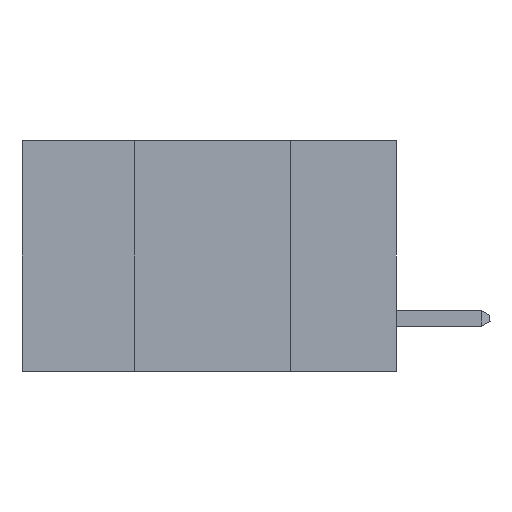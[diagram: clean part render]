
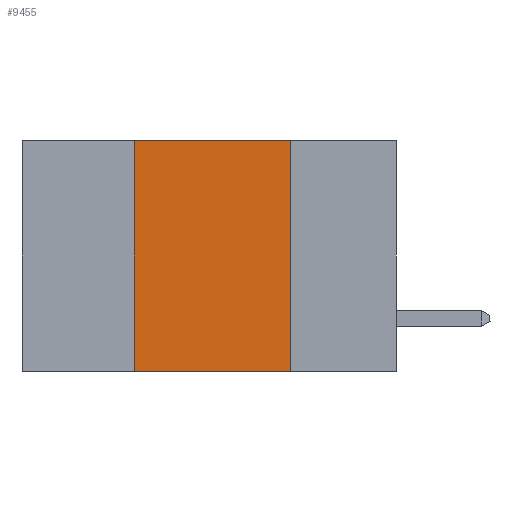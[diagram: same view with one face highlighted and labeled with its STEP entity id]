
A CAD part, left-side view. The second image highlights one B-rep face of the part: STEP entity #9455.
In plain terms, the highlighted planar face has unit normal (-1, 0, 0).
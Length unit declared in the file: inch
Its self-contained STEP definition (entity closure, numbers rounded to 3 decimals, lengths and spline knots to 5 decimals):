
#525 = CARTESIAN_POINT ( 'NONE',  ( 0., 0.17, 0. ) ) ;
#1495 = LINE ( 'NONE', #3169, #6757 ) ;
#2594 = DIRECTION ( 'NONE',  ( 0., 0., -1. ) ) ;
#2927 = CARTESIAN_POINT ( 'NONE',  ( 0., 0.42, -0.37 ) ) ;
#3167 = DIRECTION ( 'NONE',  ( 0., 0., -1. ) ) ;
#3169 = CARTESIAN_POINT ( 'NONE',  ( 0., 0.6, -0.37 ) ) ;
#3229 = AXIS2_PLACEMENT_3D ( 'NONE', #3696, #4717, #2594 ) ;
#3696 = CARTESIAN_POINT ( 'NONE',  ( 0., 0.6, 0. ) ) ;
#3770 = ORIENTED_EDGE ( 'NONE', *, *, #10901, .F. ) ;
#3911 = LINE ( 'NONE', #11110, #5869 ) ;
#4228 = DIRECTION ( 'NONE',  ( 0., -1., 0. ) ) ;
#4269 = CARTESIAN_POINT ( 'NONE',  ( 0., 0.17, 0. ) ) ;
#4399 = VECTOR ( 'NONE', #5413, 39.37008 ) ;
#4717 = DIRECTION ( 'NONE',  ( 1., 0., 0. ) ) ;
#4893 = LINE ( 'NONE', #7437, #4399 ) ;
#5028 = ORIENTED_EDGE ( 'NONE', *, *, #7295, .F. ) ;
#5382 = VERTEX_POINT ( 'NONE', #8426 ) ;
#5413 = DIRECTION ( 'NONE',  ( 0., -1., 0. ) ) ;
#5467 = EDGE_LOOP ( 'NONE', ( #8746, #5028, #3770, #12187 ) ) ;
#5651 = VERTEX_POINT ( 'NONE', #5855 ) ;
#5855 = CARTESIAN_POINT ( 'NONE',  ( 0., 0.17, -0.37 ) ) ;
#5869 = VECTOR ( 'NONE', #8908, 39.37008 ) ;
#6513 = LINE ( 'NONE', #4269, #6859 ) ;
#6757 = VECTOR ( 'NONE', #4228, 39.37008 ) ;
#6775 = PLANE ( 'NONE',  #3229 ) ;
#6859 = VECTOR ( 'NONE', #3167, 39.37008 ) ;
#7295 = EDGE_CURVE ( 'NONE', #5382, #12162, #4893, .T. ) ;
#7437 = CARTESIAN_POINT ( 'NONE',  ( 0., 0.6, 0. ) ) ;
#7615 = VERTEX_POINT ( 'NONE', #2927 ) ;
#8402 = FACE_OUTER_BOUND ( 'NONE', #5467, .T. ) ;
#8426 = CARTESIAN_POINT ( 'NONE',  ( 0., 0.42, 0. ) ) ;
#8746 = ORIENTED_EDGE ( 'NONE', *, *, #11843, .F. ) ;
#8908 = DIRECTION ( 'NONE',  ( 0., 0., 1. ) ) ;
#9115 = EDGE_CURVE ( 'NONE', #7615, #5651, #1495, .T. ) ;
#9455 = ADVANCED_FACE ( 'NONE', ( #8402 ), #6775, .F. ) ;
#10901 = EDGE_CURVE ( 'NONE', #7615, #5382, #3911, .T. ) ;
#11110 = CARTESIAN_POINT ( 'NONE',  ( 0., 0.42, 0. ) ) ;
#11843 = EDGE_CURVE ( 'NONE', #12162, #5651, #6513, .T. ) ;
#12162 = VERTEX_POINT ( 'NONE', #525 ) ;
#12187 = ORIENTED_EDGE ( 'NONE', *, *, #9115, .T. ) ;
